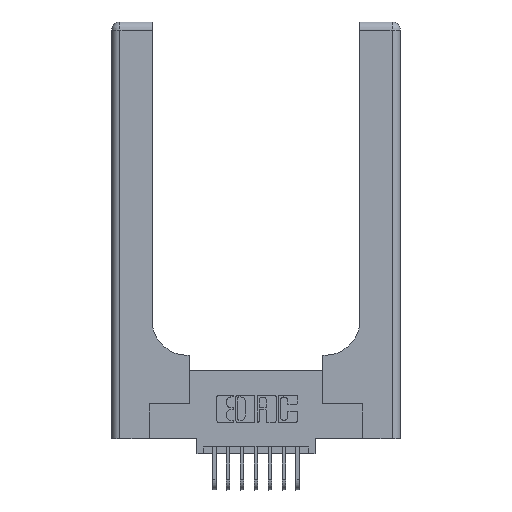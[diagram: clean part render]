
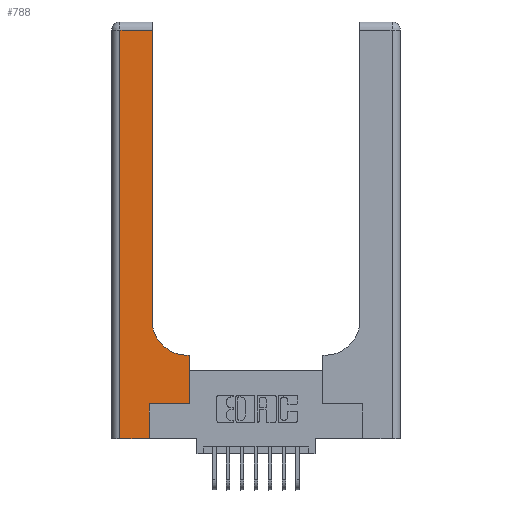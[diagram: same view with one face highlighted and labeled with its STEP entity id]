
A CAD part, top view. The second image highlights one B-rep face of the part: STEP entity #788.
In plain terms, the highlighted planar face has unit normal (0, 0, 1).
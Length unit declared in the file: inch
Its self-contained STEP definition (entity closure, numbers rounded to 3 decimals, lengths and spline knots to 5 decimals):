
#123 = EDGE_CURVE ( 'NONE', #1450, #13014, #13223, .T. ) ;
#527 = VECTOR ( 'NONE', #16344, 39.37008 ) ;
#614 = VERTEX_POINT ( 'NONE', #3269 ) ;
#788 = ADVANCED_FACE ( 'NONE', ( #1397 ), #4072, .F. ) ;
#1180 = CARTESIAN_POINT ( 'NONE',  ( 0., 2.94, 0.37 ) ) ;
#1397 = FACE_OUTER_BOUND ( 'NONE', #3967, .T. ) ;
#1450 = VERTEX_POINT ( 'NONE', #11318 ) ;
#1600 = AXIS2_PLACEMENT_3D ( 'NONE', #15804, #7925, #17116 ) ;
#1740 = EDGE_CURVE ( 'NONE', #13014, #614, #5352, .T. ) ;
#2053 = DIRECTION ( 'NONE',  ( -1., 0., 0. ) ) ;
#2071 = CARTESIAN_POINT ( 'NONE',  ( 0.269, 0., 0.37 ) ) ;
#2165 = DIRECTION ( 'NONE',  ( 0., 1., 0. ) ) ;
#2183 = DIRECTION ( 'NONE',  ( 0., 0., -1. ) ) ;
#2563 = DIRECTION ( 'NONE',  ( -1., 0., 0. ) ) ;
#2913 = DIRECTION ( 'NONE',  ( -1., 0., 0. ) ) ;
#3269 = CARTESIAN_POINT ( 'NONE',  ( 0.5585, 0.25, 0.37 ) ) ;
#3315 = EDGE_CURVE ( 'NONE', #7298, #8488, #8428, .T. ) ;
#3325 = EDGE_CURVE ( 'NONE', #4880, #13211, #4481, .T. ) ;
#3478 = VECTOR ( 'NONE', #2913, 39.37008 ) ;
#3556 = ORIENTED_EDGE ( 'NONE', *, *, #1740, .T. ) ;
#3967 = EDGE_LOOP ( 'NONE', ( #9349, #16342, #16744, #10176, #13641, #3556, #10592, #7488, #14463 ) ) ;
#4072 = PLANE ( 'NONE',  #9795 ) ;
#4123 = LINE ( 'NONE', #8470, #527 ) ;
#4481 = LINE ( 'NONE', #13592, #14149 ) ;
#4782 = CARTESIAN_POINT ( 'NONE',  ( 0., 3., 0.37 ) ) ;
#4880 = VERTEX_POINT ( 'NONE', #13072 ) ;
#5352 = LINE ( 'NONE', #11535, #15041 ) ;
#5462 = CARTESIAN_POINT ( 'NONE',  ( 0.2915, 3., 0.37 ) ) ;
#5702 = CARTESIAN_POINT ( 'NONE',  ( 0.5415, 0.6, 0.37 ) ) ;
#6235 = VECTOR ( 'NONE', #2165, 39.37008 ) ;
#6558 = VERTEX_POINT ( 'NONE', #5702 ) ;
#6999 = LINE ( 'NONE', #16066, #3478 ) ;
#7200 = DIRECTION ( 'NONE',  ( 0., 1., 0. ) ) ;
#7298 = VERTEX_POINT ( 'NONE', #9045 ) ;
#7488 = ORIENTED_EDGE ( 'NONE', *, *, #14859, .T. ) ;
#7641 = VECTOR ( 'NONE', #11055, 39.37008 ) ;
#7668 = EDGE_CURVE ( 'NONE', #13211, #1450, #11551, .T. ) ;
#7713 = EDGE_CURVE ( 'NONE', #614, #10496, #4123, .T. ) ;
#7925 = DIRECTION ( 'NONE',  ( 0., 0., -1. ) ) ;
#8021 = LINE ( 'NONE', #1180, #14579 ) ;
#8085 = EDGE_CURVE ( 'NONE', #6558, #7298, #8866, .T. ) ;
#8428 = LINE ( 'NONE', #5462, #15400 ) ;
#8470 = CARTESIAN_POINT ( 'NONE',  ( 0.5585, 0.25, 0.37 ) ) ;
#8488 = VERTEX_POINT ( 'NONE', #13823 ) ;
#8641 = EDGE_CURVE ( 'NONE', #8488, #4880, #8021, .T. ) ;
#8866 = CIRCLE ( 'NONE', #1600, 0.25 ) ;
#9045 = CARTESIAN_POINT ( 'NONE',  ( 0.2915, 0.85, 0.37 ) ) ;
#9349 = ORIENTED_EDGE ( 'NONE', *, *, #3315, .T. ) ;
#9733 = CARTESIAN_POINT ( 'NONE',  ( 0., 0., 0.37 ) ) ;
#9795 = AXIS2_PLACEMENT_3D ( 'NONE', #4782, #2183, #2053 ) ;
#10040 = CARTESIAN_POINT ( 'NONE',  ( 0.5585, 0.6, 0.37 ) ) ;
#10176 = ORIENTED_EDGE ( 'NONE', *, *, #7668, .T. ) ;
#10496 = VERTEX_POINT ( 'NONE', #10040 ) ;
#10592 = ORIENTED_EDGE ( 'NONE', *, *, #7713, .T. ) ;
#11055 = DIRECTION ( 'NONE',  ( 1., 0., 0. ) ) ;
#11318 = CARTESIAN_POINT ( 'NONE',  ( 0.269, 0., 0.37 ) ) ;
#11535 = CARTESIAN_POINT ( 'NONE',  ( 0.269, 0.25, 0.37 ) ) ;
#11551 = LINE ( 'NONE', #9733, #7641 ) ;
#12024 = DIRECTION ( 'NONE',  ( 1., 0., 0. ) ) ;
#13014 = VERTEX_POINT ( 'NONE', #16749 ) ;
#13072 = CARTESIAN_POINT ( 'NONE',  ( 0.06, 2.94, 0.37 ) ) ;
#13211 = VERTEX_POINT ( 'NONE', #17192 ) ;
#13223 = LINE ( 'NONE', #2071, #6235 ) ;
#13592 = CARTESIAN_POINT ( 'NONE',  ( 0.06, 3., 0.37 ) ) ;
#13641 = ORIENTED_EDGE ( 'NONE', *, *, #123, .T. ) ;
#13823 = CARTESIAN_POINT ( 'NONE',  ( 0.2915, 2.94, 0.37 ) ) ;
#14149 = VECTOR ( 'NONE', #15742, 39.37008 ) ;
#14463 = ORIENTED_EDGE ( 'NONE', *, *, #8085, .T. ) ;
#14579 = VECTOR ( 'NONE', #2563, 39.37008 ) ;
#14859 = EDGE_CURVE ( 'NONE', #10496, #6558, #6999, .T. ) ;
#15041 = VECTOR ( 'NONE', #12024, 39.37008 ) ;
#15400 = VECTOR ( 'NONE', #7200, 39.37008 ) ;
#15742 = DIRECTION ( 'NONE',  ( 0., -1., 0. ) ) ;
#15804 = CARTESIAN_POINT ( 'NONE',  ( 0.5415, 0.85, 0.37 ) ) ;
#16066 = CARTESIAN_POINT ( 'NONE',  ( 0.2915, 0.6, 0.37 ) ) ;
#16342 = ORIENTED_EDGE ( 'NONE', *, *, #8641, .T. ) ;
#16344 = DIRECTION ( 'NONE',  ( 0., 1., 0. ) ) ;
#16744 = ORIENTED_EDGE ( 'NONE', *, *, #3325, .T. ) ;
#16749 = CARTESIAN_POINT ( 'NONE',  ( 0.269, 0.25, 0.37 ) ) ;
#17116 = DIRECTION ( 'NONE',  ( 1., 0., 0. ) ) ;
#17192 = CARTESIAN_POINT ( 'NONE',  ( 0.06, 0., 0.37 ) ) ;
